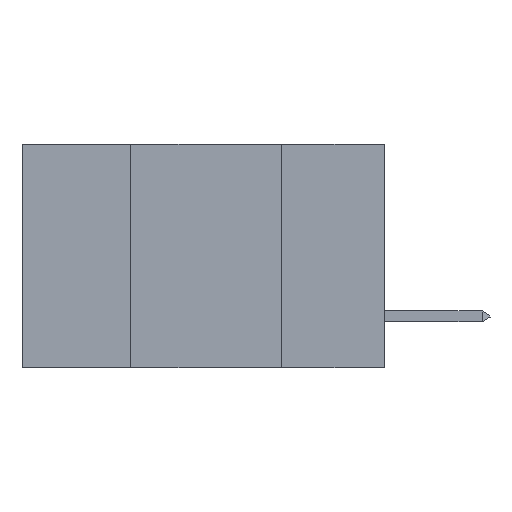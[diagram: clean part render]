
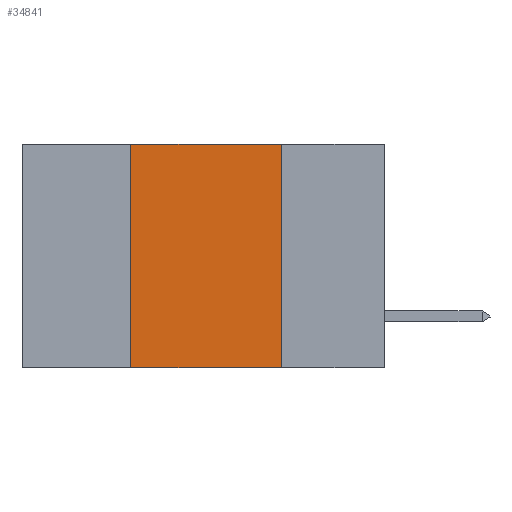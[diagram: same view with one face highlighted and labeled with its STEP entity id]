
A CAD part, left-side view. The second image highlights one B-rep face of the part: STEP entity #34841.
In plain terms, the highlighted planar face has unit normal (-1, 0, 0).
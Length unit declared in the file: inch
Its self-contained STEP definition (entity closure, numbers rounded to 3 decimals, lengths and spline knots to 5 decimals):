
#4325 = FACE_OUTER_BOUND ( 'NONE', #15246, .T. ) ;
#4506 = EDGE_CURVE ( 'NONE', #7263, #29394, #44013, .T. ) ;
#5074 = VERTEX_POINT ( 'NONE', #15742 ) ;
#6606 = CARTESIAN_POINT ( 'NONE',  ( 0., 0.6, 0. ) ) ;
#7263 = VERTEX_POINT ( 'NONE', #30767 ) ;
#8512 = DIRECTION ( 'NONE',  ( 0., -1., 0. ) ) ;
#10094 = ORIENTED_EDGE ( 'NONE', *, *, #31317, .T. ) ;
#12569 = VECTOR ( 'NONE', #43957, 39.37008 ) ;
#14158 = CARTESIAN_POINT ( 'NONE',  ( 0., 0.6, 0. ) ) ;
#14856 = CARTESIAN_POINT ( 'NONE',  ( 0., 0.17, 0. ) ) ;
#15123 = LINE ( 'NONE', #50024, #12569 ) ;
#15246 = EDGE_LOOP ( 'NONE', ( #25810, #25871, #26561, #10094 ) ) ;
#15370 = AXIS2_PLACEMENT_3D ( 'NONE', #14158, #41651, #18353 ) ;
#15742 = CARTESIAN_POINT ( 'NONE',  ( 0., 0.17, -0.37 ) ) ;
#16168 = EDGE_CURVE ( 'NONE', #26844, #7263, #33087, .T. ) ;
#18353 = DIRECTION ( 'NONE',  ( 0., 0., -1. ) ) ;
#20000 = EDGE_CURVE ( 'NONE', #29394, #5074, #15123, .T. ) ;
#21013 = CARTESIAN_POINT ( 'NONE',  ( 0., 0.42, 0. ) ) ;
#22158 = CARTESIAN_POINT ( 'NONE',  ( 0., 0.42, -0.37 ) ) ;
#23312 = PLANE ( 'NONE',  #15370 ) ;
#23401 = VECTOR ( 'NONE', #41501, 39.37008 ) ;
#23810 = DIRECTION ( 'NONE',  ( 0., 0., 1. ) ) ;
#25810 = ORIENTED_EDGE ( 'NONE', *, *, #20000, .F. ) ;
#25871 = ORIENTED_EDGE ( 'NONE', *, *, #4506, .F. ) ;
#26561 = ORIENTED_EDGE ( 'NONE', *, *, #16168, .F. ) ;
#26844 = VERTEX_POINT ( 'NONE', #22158 ) ;
#27710 = CARTESIAN_POINT ( 'NONE',  ( 0., 0.6, -0.37 ) ) ;
#29394 = VERTEX_POINT ( 'NONE', #14856 ) ;
#30767 = CARTESIAN_POINT ( 'NONE',  ( 0., 0.42, 0. ) ) ;
#31317 = EDGE_CURVE ( 'NONE', #26844, #5074, #37300, .T. ) ;
#33087 = LINE ( 'NONE', #21013, #34917 ) ;
#34841 = ADVANCED_FACE ( 'NONE', ( #4325 ), #23312, .F. ) ;
#34917 = VECTOR ( 'NONE', #23810, 39.37008 ) ;
#37300 = LINE ( 'NONE', #27710, #43902 ) ;
#41501 = DIRECTION ( 'NONE',  ( 0., -1., 0. ) ) ;
#41651 = DIRECTION ( 'NONE',  ( 1., 0., 0. ) ) ;
#43902 = VECTOR ( 'NONE', #8512, 39.37008 ) ;
#43957 = DIRECTION ( 'NONE',  ( 0., 0., -1. ) ) ;
#44013 = LINE ( 'NONE', #6606, #23401 ) ;
#50024 = CARTESIAN_POINT ( 'NONE',  ( 0., 0.17, 0. ) ) ;
